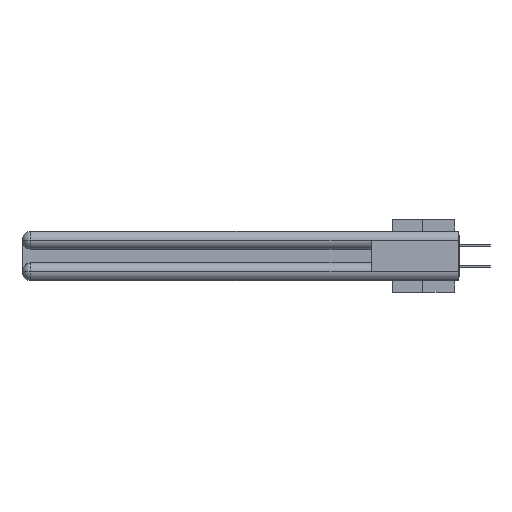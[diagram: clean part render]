
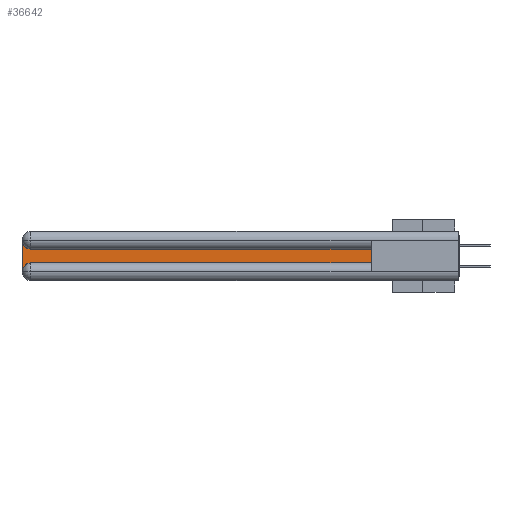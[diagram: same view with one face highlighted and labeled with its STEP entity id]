
A CAD part, left-side view. The second image highlights one B-rep face of the part: STEP entity #36642.
In plain terms, the highlighted planar face has unit normal (-1, 0, 0).
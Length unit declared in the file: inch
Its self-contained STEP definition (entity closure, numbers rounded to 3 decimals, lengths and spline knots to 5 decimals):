
#15 = EDGE_CURVE ( 'NONE', #12797, #29449, #14097, .T. ) ;
#141 = EDGE_CURVE ( 'NONE', #23529, #12797, #32410, .T. ) ;
#976 = ORIENTED_EDGE ( 'NONE', *, *, #47764, .T. ) ;
#1472 = ORIENTED_EDGE ( 'NONE', *, *, #15, .T. ) ;
#1903 = ORIENTED_EDGE ( 'NONE', *, *, #43621, .T. ) ;
#2291 = AXIS2_PLACEMENT_3D ( 'NONE', #12266, #16235, #34461 ) ;
#5469 = CARTESIAN_POINT ( 'NONE',  ( 0.075, 2.94, -0.0625 ) ) ;
#5748 = FACE_OUTER_BOUND ( 'NONE', #43888, .T. ) ;
#6419 = VECTOR ( 'NONE', #36277, 39.37008 ) ;
#7132 = DIRECTION ( 'NONE',  ( 0., 0., -1. ) ) ;
#8785 = DIRECTION ( 'NONE',  ( 1., 0., 0. ) ) ;
#9615 = VECTOR ( 'NONE', #45764, 39.37008 ) ;
#11864 = CARTESIAN_POINT ( 'NONE',  ( 0.075, 0.6, -0.1225 ) ) ;
#12266 = CARTESIAN_POINT ( 'NONE',  ( 0.075, 2.94, -0.2775 ) ) ;
#12797 = VERTEX_POINT ( 'NONE', #11864 ) ;
#14097 = LINE ( 'NONE', #31294, #43660 ) ;
#15169 = VERTEX_POINT ( 'NONE', #17118 ) ;
#16235 = DIRECTION ( 'NONE',  ( 1., 0., 0. ) ) ;
#17118 = CARTESIAN_POINT ( 'NONE',  ( 0.075, 3., -0.0625 ) ) ;
#17577 = CARTESIAN_POINT ( 'NONE',  ( 0.075, 0.6, -0.2175 ) ) ;
#18876 = CARTESIAN_POINT ( 'NONE',  ( 0.075, 3., -0.2175 ) ) ;
#19325 = CARTESIAN_POINT ( 'NONE',  ( 0.075, 0.6, -0.2175 ) ) ;
#19689 = PLANE ( 'NONE',  #26944 ) ;
#20264 = CARTESIAN_POINT ( 'NONE',  ( 0.075, 2.94, -0.1225 ) ) ;
#22741 = CIRCLE ( 'NONE', #2291, 0.06 ) ;
#23529 = VERTEX_POINT ( 'NONE', #25112 ) ;
#23617 = AXIS2_PLACEMENT_3D ( 'NONE', #5469, #36070, #31584 ) ;
#25048 = VECTOR ( 'NONE', #7132, 39.37008 ) ;
#25112 = CARTESIAN_POINT ( 'NONE',  ( 0.075, 0.6, -0.2175 ) ) ;
#26512 = EDGE_CURVE ( 'NONE', #34244, #44237, #22741, .T. ) ;
#26944 = AXIS2_PLACEMENT_3D ( 'NONE', #31392, #8785, #31088 ) ;
#29449 = VERTEX_POINT ( 'NONE', #20264 ) ;
#31088 = DIRECTION ( 'NONE',  ( 0., 0., -1. ) ) ;
#31294 = CARTESIAN_POINT ( 'NONE',  ( 0.075, 0.6, -0.1225 ) ) ;
#31359 = ORIENTED_EDGE ( 'NONE', *, *, #26512, .T. ) ;
#31392 = CARTESIAN_POINT ( 'NONE',  ( 0.075, 3., -0.1225 ) ) ;
#31584 = DIRECTION ( 'NONE',  ( 0., 0., -1. ) ) ;
#32410 = LINE ( 'NONE', #17577, #6419 ) ;
#33111 = CARTESIAN_POINT ( 'NONE',  ( 0.075, 2.94, -0.2175 ) ) ;
#34244 = VERTEX_POINT ( 'NONE', #40004 ) ;
#34461 = DIRECTION ( 'NONE',  ( 0., 0., -1. ) ) ;
#36070 = DIRECTION ( 'NONE',  ( 1., 0., 0. ) ) ;
#36277 = DIRECTION ( 'NONE',  ( 0., 0., 1. ) ) ;
#36642 = ADVANCED_FACE ( 'NONE', ( #5748 ), #19689, .F. ) ;
#39196 = LINE ( 'NONE', #18876, #25048 ) ;
#40004 = CARTESIAN_POINT ( 'NONE',  ( 0.075, 3., -0.2775 ) ) ;
#41515 = ORIENTED_EDGE ( 'NONE', *, *, #48139, .T. ) ;
#41587 = CIRCLE ( 'NONE', #23617, 0.06 ) ;
#43621 = EDGE_CURVE ( 'NONE', #15169, #34244, #39196, .T. ) ;
#43660 = VECTOR ( 'NONE', #44065, 39.37008 ) ;
#43888 = EDGE_LOOP ( 'NONE', ( #1472, #976, #1903, #31359, #41515, #48804 ) ) ;
#43948 = LINE ( 'NONE', #19325, #9615 ) ;
#44065 = DIRECTION ( 'NONE',  ( 0., 1., 0. ) ) ;
#44237 = VERTEX_POINT ( 'NONE', #33111 ) ;
#45764 = DIRECTION ( 'NONE',  ( 0., -1., 0. ) ) ;
#47764 = EDGE_CURVE ( 'NONE', #29449, #15169, #41587, .T. ) ;
#48139 = EDGE_CURVE ( 'NONE', #44237, #23529, #43948, .T. ) ;
#48804 = ORIENTED_EDGE ( 'NONE', *, *, #141, .T. ) ;
